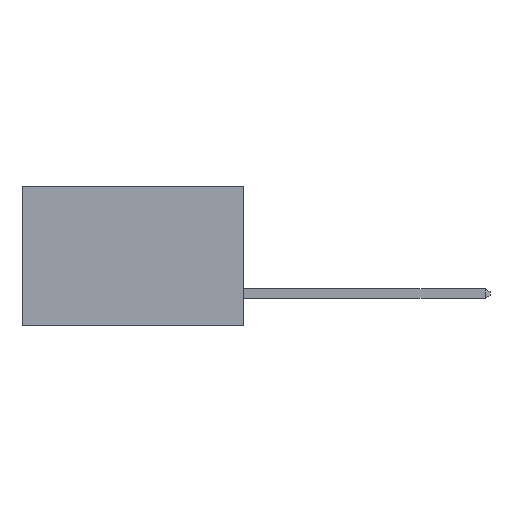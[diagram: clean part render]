
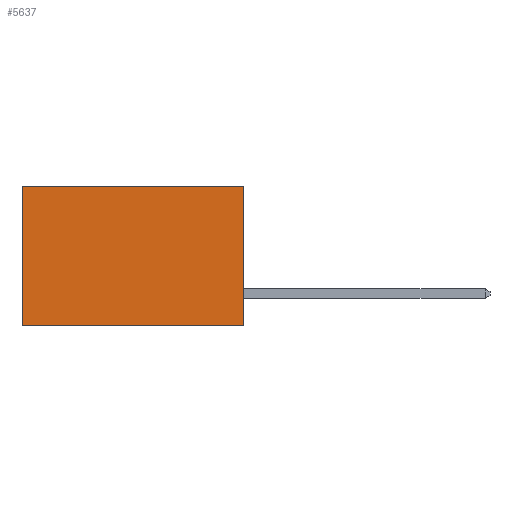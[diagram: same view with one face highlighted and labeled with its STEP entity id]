
A CAD part, left-side view. The second image highlights one B-rep face of the part: STEP entity #5637.
In plain terms, the highlighted planar face has unit normal (-1, 0, 0).
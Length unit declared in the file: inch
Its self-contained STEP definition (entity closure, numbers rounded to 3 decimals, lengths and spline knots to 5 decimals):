
#206 = ORIENTED_EDGE ( 'NONE', *, *, #4127, .T. ) ;
#521 = FACE_OUTER_BOUND ( 'NONE', #3796, .T. ) ;
#1255 = ORIENTED_EDGE ( 'NONE', *, *, #8288, .T. ) ;
#1280 = EDGE_CURVE ( 'NONE', #3069, #1366, #7568, .T. ) ;
#1366 = VERTEX_POINT ( 'NONE', #6545 ) ;
#1432 = VERTEX_POINT ( 'NONE', #5707 ) ;
#1438 = ORIENTED_EDGE ( 'NONE', *, *, #2875, .F. ) ;
#1645 = DIRECTION ( 'NONE',  ( 0., 0., -1. ) ) ;
#1917 = VECTOR ( 'NONE', #3294, 39.37008 ) ;
#2337 = CARTESIAN_POINT ( 'NONE',  ( 0.277, 0., -0.37 ) ) ;
#2358 = DIRECTION ( 'NONE',  ( 0., 0., -1. ) ) ;
#2408 = DIRECTION ( 'NONE',  ( 1., 0., 0. ) ) ;
#2433 = CARTESIAN_POINT ( 'NONE',  ( 0.277, 0., -0.37 ) ) ;
#2456 = PLANE ( 'NONE',  #8266 ) ;
#2584 = VECTOR ( 'NONE', #2846, 39.37008 ) ;
#2846 = DIRECTION ( 'NONE',  ( 0., 1., 0. ) ) ;
#2875 = EDGE_CURVE ( 'NONE', #1432, #3069, #7242, .T. ) ;
#3069 = VERTEX_POINT ( 'NONE', #5944 ) ;
#3294 = DIRECTION ( 'NONE',  ( 0., 1., 0. ) ) ;
#3402 = CARTESIAN_POINT ( 'NONE',  ( 0.277, 0., 0. ) ) ;
#3711 = CARTESIAN_POINT ( 'NONE',  ( 0.277, 0.59, 0. ) ) ;
#3796 = EDGE_LOOP ( 'NONE', ( #206, #5192, #1438, #1255 ) ) ;
#4127 = EDGE_CURVE ( 'NONE', #8884, #1366, #7848, .T. ) ;
#5192 = ORIENTED_EDGE ( 'NONE', *, *, #1280, .F. ) ;
#5462 = VECTOR ( 'NONE', #1645, 39.37008 ) ;
#5528 = DIRECTION ( 'NONE',  ( 0., 0., -1. ) ) ;
#5637 = ADVANCED_FACE ( 'NONE', ( #521 ), #2456, .F. ) ;
#5674 = CARTESIAN_POINT ( 'NONE',  ( 0.277, 0.59, -0.37 ) ) ;
#5707 = CARTESIAN_POINT ( 'NONE',  ( 0.277, 0., 0. ) ) ;
#5944 = CARTESIAN_POINT ( 'NONE',  ( 0.277, 0., -0.37 ) ) ;
#6545 = CARTESIAN_POINT ( 'NONE',  ( 0.277, 0.59, -0.37 ) ) ;
#7047 = CARTESIAN_POINT ( 'NONE',  ( 0.277, 0., -0.37 ) ) ;
#7242 = LINE ( 'NONE', #2337, #5462 ) ;
#7380 = LINE ( 'NONE', #3402, #1917 ) ;
#7568 = LINE ( 'NONE', #7047, #2584 ) ;
#7848 = LINE ( 'NONE', #5674, #8028 ) ;
#8028 = VECTOR ( 'NONE', #5528, 39.37008 ) ;
#8266 = AXIS2_PLACEMENT_3D ( 'NONE', #2433, #2408, #2358 ) ;
#8288 = EDGE_CURVE ( 'NONE', #1432, #8884, #7380, .T. ) ;
#8884 = VERTEX_POINT ( 'NONE', #3711 ) ;
